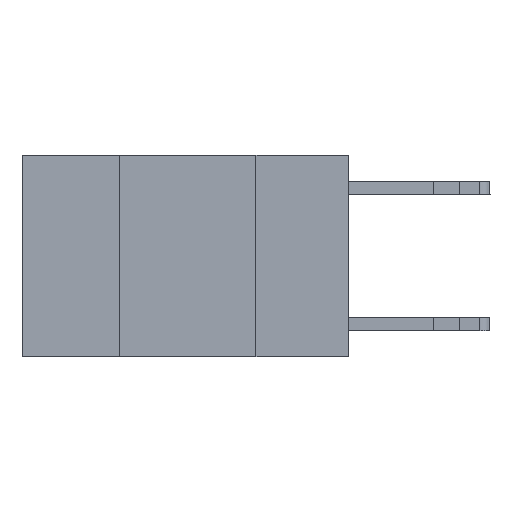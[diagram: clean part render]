
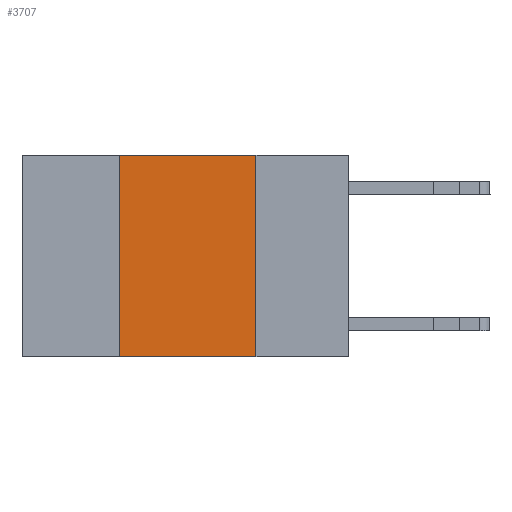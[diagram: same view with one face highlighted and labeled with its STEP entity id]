
A CAD part, left-side view. The second image highlights one B-rep face of the part: STEP entity #3707.
In plain terms, the highlighted planar face has unit normal (-1, 0, 0).
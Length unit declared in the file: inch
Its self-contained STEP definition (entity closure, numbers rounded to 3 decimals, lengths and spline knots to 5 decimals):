
#182 = CARTESIAN_POINT ( 'NONE',  ( 0., 0.42, 0. ) ) ;
#1182 = VERTEX_POINT ( 'NONE', #6288 ) ;
#1929 = ORIENTED_EDGE ( 'NONE', *, *, #4463, .F. ) ;
#2379 = DIRECTION ( 'NONE',  ( 0., 0., -1. ) ) ;
#2596 = CARTESIAN_POINT ( 'NONE',  ( 0., 0.42, -0.37 ) ) ;
#2700 = EDGE_CURVE ( 'NONE', #14136, #1182, #8057, .T. ) ;
#2800 = ORIENTED_EDGE ( 'NONE', *, *, #15739, .F. ) ;
#3707 = ADVANCED_FACE ( 'NONE', ( #6800 ), #4872, .F. ) ;
#4463 = EDGE_CURVE ( 'NONE', #6970, #6002, #12897, .T. ) ;
#4471 = CARTESIAN_POINT ( 'NONE',  ( 0., 0.6, 0. ) ) ;
#4628 = VECTOR ( 'NONE', #11148, 39.37008 ) ;
#4872 = PLANE ( 'NONE',  #5057 ) ;
#5057 = AXIS2_PLACEMENT_3D ( 'NONE', #7562, #16826, #8875 ) ;
#6002 = VERTEX_POINT ( 'NONE', #12999 ) ;
#6288 = CARTESIAN_POINT ( 'NONE',  ( 0., 0.42, 0. ) ) ;
#6800 = FACE_OUTER_BOUND ( 'NONE', #11834, .T. ) ;
#6970 = VERTEX_POINT ( 'NONE', #16140 ) ;
#7562 = CARTESIAN_POINT ( 'NONE',  ( 0., 0.6, 0. ) ) ;
#8057 = LINE ( 'NONE', #182, #11228 ) ;
#8875 = DIRECTION ( 'NONE',  ( 0., 0., -1. ) ) ;
#11148 = DIRECTION ( 'NONE',  ( 0., -1., 0. ) ) ;
#11228 = VECTOR ( 'NONE', #12209, 39.37008 ) ;
#11834 = EDGE_LOOP ( 'NONE', ( #1929, #2800, #12456, #13673 ) ) ;
#12209 = DIRECTION ( 'NONE',  ( 0., 0., 1. ) ) ;
#12227 = LINE ( 'NONE', #4471, #4628 ) ;
#12456 = ORIENTED_EDGE ( 'NONE', *, *, #2700, .F. ) ;
#12491 = VECTOR ( 'NONE', #2379, 39.37008 ) ;
#12897 = LINE ( 'NONE', #13079, #12491 ) ;
#12999 = CARTESIAN_POINT ( 'NONE',  ( 0., 0.17, -0.37 ) ) ;
#13079 = CARTESIAN_POINT ( 'NONE',  ( 0., 0.17, 0. ) ) ;
#13673 = ORIENTED_EDGE ( 'NONE', *, *, #16385, .T. ) ;
#14136 = VERTEX_POINT ( 'NONE', #2596 ) ;
#15053 = VECTOR ( 'NONE', #16485, 39.37008 ) ;
#15181 = CARTESIAN_POINT ( 'NONE',  ( 0., 0.6, -0.37 ) ) ;
#15477 = LINE ( 'NONE', #15181, #15053 ) ;
#15739 = EDGE_CURVE ( 'NONE', #1182, #6970, #12227, .T. ) ;
#16140 = CARTESIAN_POINT ( 'NONE',  ( 0., 0.17, 0. ) ) ;
#16385 = EDGE_CURVE ( 'NONE', #14136, #6002, #15477, .T. ) ;
#16485 = DIRECTION ( 'NONE',  ( 0., -1., 0. ) ) ;
#16826 = DIRECTION ( 'NONE',  ( 1., 0., 0. ) ) ;
